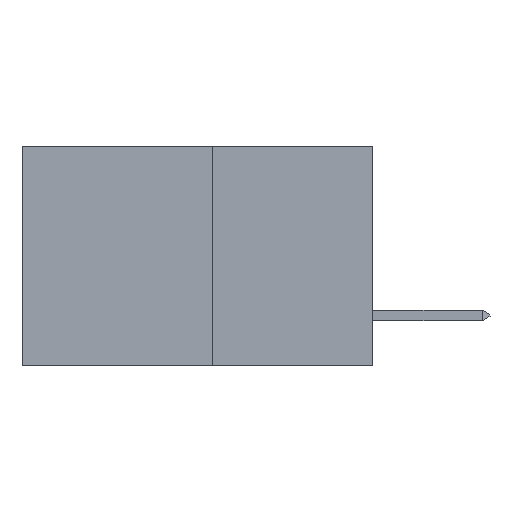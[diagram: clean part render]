
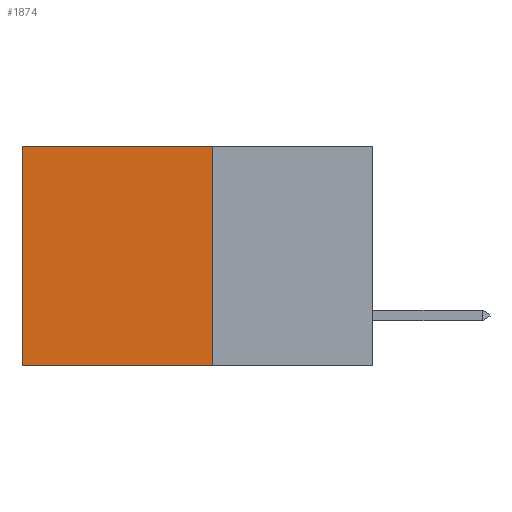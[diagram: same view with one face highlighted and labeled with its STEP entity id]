
A CAD part, left-side view. The second image highlights one B-rep face of the part: STEP entity #1874.
In plain terms, the highlighted planar face has unit normal (-1, 0, 0).
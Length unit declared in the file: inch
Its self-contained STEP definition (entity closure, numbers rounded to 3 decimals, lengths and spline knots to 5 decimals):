
#124 = CARTESIAN_POINT ( 'NONE',  ( 0.277, 0.27, -0.37 ) ) ;
#135 = CARTESIAN_POINT ( 'NONE',  ( 0.277, 0.27, -0.37 ) ) ;
#251 = LINE ( 'NONE', #2988, #3877 ) ;
#526 = ORIENTED_EDGE ( 'NONE', *, *, #4940, .F. ) ;
#772 = VECTOR ( 'NONE', #2669, 39.37008 ) ;
#966 = DIRECTION ( 'NONE',  ( 0., 1., 0. ) ) ;
#1742 = EDGE_CURVE ( 'NONE', #7191, #5982, #6838, .T. ) ;
#1802 = EDGE_LOOP ( 'NONE', ( #6393, #526, #3059, #6495 ) ) ;
#1874 = ADVANCED_FACE ( 'NONE', ( #5776 ), #5058, .F. ) ;
#2453 = CARTESIAN_POINT ( 'NONE',  ( 0.277, 0.59, 0. ) ) ;
#2667 = VERTEX_POINT ( 'NONE', #6266 ) ;
#2669 = DIRECTION ( 'NONE',  ( 0., 1., 0. ) ) ;
#2930 = LINE ( 'NONE', #4816, #772 ) ;
#2988 = CARTESIAN_POINT ( 'NONE',  ( 0.277, 0.27, -0.37 ) ) ;
#3059 = ORIENTED_EDGE ( 'NONE', *, *, #5207, .F. ) ;
#3126 = VERTEX_POINT ( 'NONE', #135 ) ;
#3167 = CARTESIAN_POINT ( 'NONE',  ( 0.277, 0.59, -0.37 ) ) ;
#3521 = VECTOR ( 'NONE', #966, 39.37008 ) ;
#3775 = LINE ( 'NONE', #124, #3521 ) ;
#3822 = AXIS2_PLACEMENT_3D ( 'NONE', #5524, #8382, #8799 ) ;
#3877 = VECTOR ( 'NONE', #4241, 39.37008 ) ;
#4241 = DIRECTION ( 'NONE',  ( 0., 0., -1. ) ) ;
#4323 = DIRECTION ( 'NONE',  ( 0., 0., -1. ) ) ;
#4816 = CARTESIAN_POINT ( 'NONE',  ( 0.277, 0.27, 0. ) ) ;
#4940 = EDGE_CURVE ( 'NONE', #3126, #5982, #3775, .T. ) ;
#5058 = PLANE ( 'NONE',  #3822 ) ;
#5064 = EDGE_CURVE ( 'NONE', #2667, #7191, #2930, .T. ) ;
#5207 = EDGE_CURVE ( 'NONE', #2667, #3126, #251, .T. ) ;
#5524 = CARTESIAN_POINT ( 'NONE',  ( 0.277, 0.27, -0.37 ) ) ;
#5776 = FACE_OUTER_BOUND ( 'NONE', #1802, .T. ) ;
#5982 = VERTEX_POINT ( 'NONE', #6116 ) ;
#6116 = CARTESIAN_POINT ( 'NONE',  ( 0.277, 0.59, -0.37 ) ) ;
#6266 = CARTESIAN_POINT ( 'NONE',  ( 0.277, 0.27, 0. ) ) ;
#6393 = ORIENTED_EDGE ( 'NONE', *, *, #1742, .T. ) ;
#6495 = ORIENTED_EDGE ( 'NONE', *, *, #5064, .T. ) ;
#6838 = LINE ( 'NONE', #3167, #8398 ) ;
#7191 = VERTEX_POINT ( 'NONE', #2453 ) ;
#8382 = DIRECTION ( 'NONE',  ( 1., 0., 0. ) ) ;
#8398 = VECTOR ( 'NONE', #4323, 39.37008 ) ;
#8799 = DIRECTION ( 'NONE',  ( 0., 0., -1. ) ) ;
